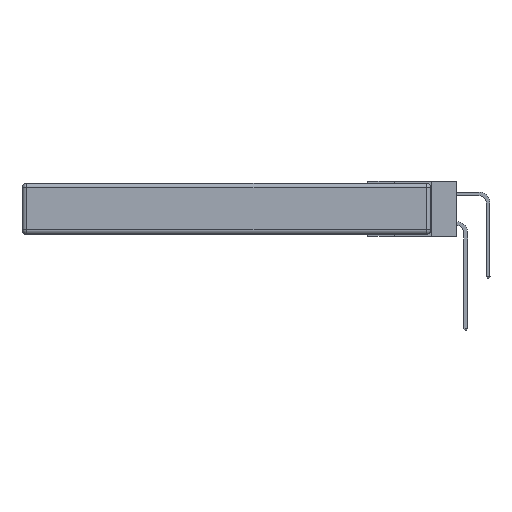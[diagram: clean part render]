
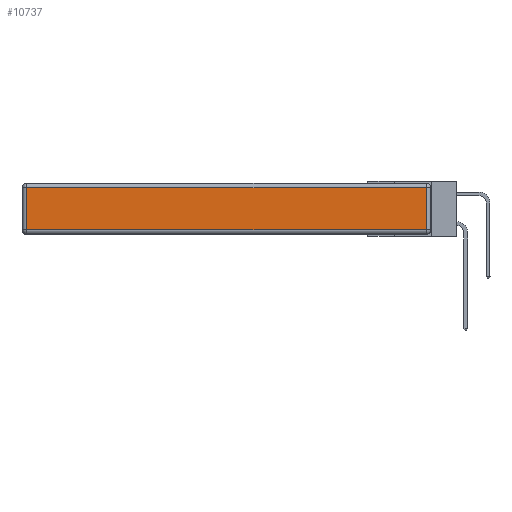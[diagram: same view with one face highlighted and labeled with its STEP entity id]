
A CAD part, left-side view. The second image highlights one B-rep face of the part: STEP entity #10737.
In plain terms, the highlighted planar face has unit normal (-1, 0, 0).
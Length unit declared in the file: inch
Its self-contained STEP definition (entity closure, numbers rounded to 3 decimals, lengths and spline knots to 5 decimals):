
#1136 = CARTESIAN_POINT ( 'NONE',  ( 0., 2.72, -0.313 ) ) ;
#1915 = CARTESIAN_POINT ( 'NONE',  ( 0., 0.03, -0.343 ) ) ;
#2433 = DIRECTION ( 'NONE',  ( 0., 1., 0. ) ) ;
#2476 = VERTEX_POINT ( 'NONE', #11793 ) ;
#3608 = ORIENTED_EDGE ( 'NONE', *, *, #17198, .T. ) ;
#3841 = PLANE ( 'NONE',  #17981 ) ;
#4509 = CARTESIAN_POINT ( 'NONE',  ( 0., 0., -0.313 ) ) ;
#4802 = VECTOR ( 'NONE', #7087, 39.37008 ) ;
#5047 = DIRECTION ( 'NONE',  ( 0., 0., 1. ) ) ;
#5371 = DIRECTION ( 'NONE',  ( -1., 0., 0. ) ) ;
#5908 = LINE ( 'NONE', #4509, #15212 ) ;
#6545 = ORIENTED_EDGE ( 'NONE', *, *, #11204, .T. ) ;
#6878 = CARTESIAN_POINT ( 'NONE',  ( 0., 0., -0.343 ) ) ;
#7087 = DIRECTION ( 'NONE',  ( 0., 0., -1. ) ) ;
#7163 = VECTOR ( 'NONE', #2433, 39.37008 ) ;
#8326 = DIRECTION ( 'NONE',  ( 0., -1., 0. ) ) ;
#10022 = LINE ( 'NONE', #10155, #4802 ) ;
#10155 = CARTESIAN_POINT ( 'NONE',  ( 0., 2.72, -0.343 ) ) ;
#10450 = ORIENTED_EDGE ( 'NONE', *, *, #16933, .T. ) ;
#10737 = ADVANCED_FACE ( 'NONE', ( #13637 ), #3841, .T. ) ;
#10797 = VERTEX_POINT ( 'NONE', #1136 ) ;
#10957 = VERTEX_POINT ( 'NONE', #12249 ) ;
#11204 = EDGE_CURVE ( 'NONE', #19258, #10957, #18188, .T. ) ;
#11793 = CARTESIAN_POINT ( 'NONE',  ( 0., 0.03, -0.313 ) ) ;
#12249 = CARTESIAN_POINT ( 'NONE',  ( 0., 2.72, -0.03 ) ) ;
#12579 = LINE ( 'NONE', #1915, #18809 ) ;
#12956 = CARTESIAN_POINT ( 'NONE',  ( 0., 0.03, -0.03 ) ) ;
#13302 = EDGE_LOOP ( 'NONE', ( #10450, #3608, #6545, #15723 ) ) ;
#13637 = FACE_OUTER_BOUND ( 'NONE', #13302, .T. ) ;
#14701 = EDGE_CURVE ( 'NONE', #10957, #10797, #10022, .T. ) ;
#15212 = VECTOR ( 'NONE', #8326, 39.37008 ) ;
#15723 = ORIENTED_EDGE ( 'NONE', *, *, #14701, .T. ) ;
#16933 = EDGE_CURVE ( 'NONE', #10797, #2476, #5908, .T. ) ;
#17198 = EDGE_CURVE ( 'NONE', #2476, #19258, #12579, .T. ) ;
#17789 = CARTESIAN_POINT ( 'NONE',  ( 0., 2.75, -0.03 ) ) ;
#17981 = AXIS2_PLACEMENT_3D ( 'NONE', #6878, #5371, #18928 ) ;
#18188 = LINE ( 'NONE', #17789, #7163 ) ;
#18809 = VECTOR ( 'NONE', #5047, 39.37008 ) ;
#18928 = DIRECTION ( 'NONE',  ( 0., 0., 1. ) ) ;
#19258 = VERTEX_POINT ( 'NONE', #12956 ) ;
